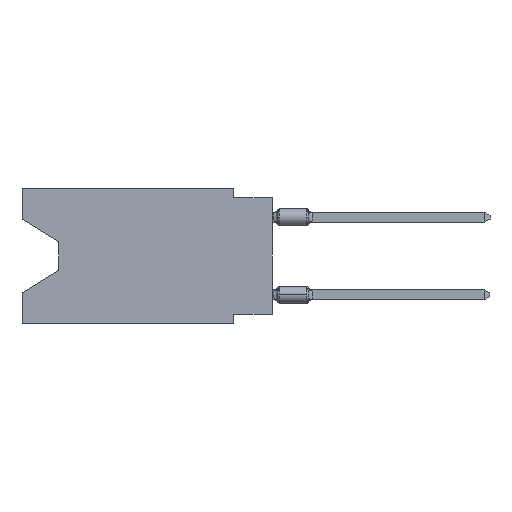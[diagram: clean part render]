
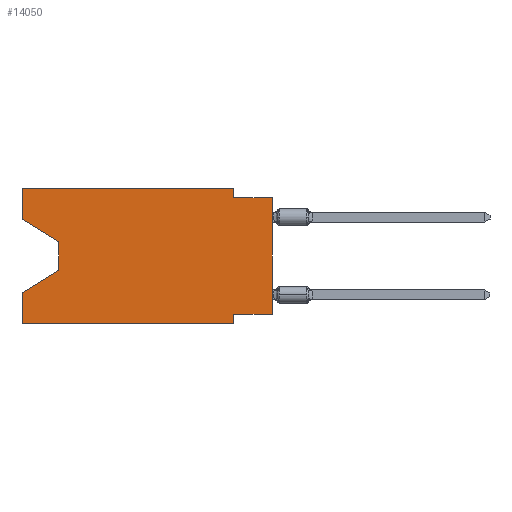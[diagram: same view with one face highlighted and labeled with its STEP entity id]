
A CAD part, left-side view. The second image highlights one B-rep face of the part: STEP entity #14050.
In plain terms, the highlighted planar face has unit normal (-1, 0, 0).
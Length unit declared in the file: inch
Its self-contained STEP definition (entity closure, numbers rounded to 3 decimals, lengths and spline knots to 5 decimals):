
#282 = CARTESIAN_POINT ( 'NONE',  ( 0., 0.1, -0.35 ) ) ;
#791 = FACE_OUTER_BOUND ( 'NONE', #29881, .T. ) ;
#947 = CARTESIAN_POINT ( 'NONE',  ( 0., 0.645, 0. ) ) ;
#1299 = LINE ( 'NONE', #24705, #29097 ) ;
#1441 = EDGE_CURVE ( 'NONE', #24950, #22444, #23115, .T. ) ;
#1586 = VERTEX_POINT ( 'NONE', #23418 ) ;
#1591 = CARTESIAN_POINT ( 'NONE',  ( 0., 0.645, 0. ) ) ;
#1623 = EDGE_CURVE ( 'NONE', #25172, #11600, #10286, .T. ) ;
#2054 = EDGE_CURVE ( 'NONE', #12673, #2710, #5565, .T. ) ;
#2333 = CARTESIAN_POINT ( 'NONE',  ( 0., 0.645, 0. ) ) ;
#2710 = VERTEX_POINT ( 'NONE', #29706 ) ;
#2850 = PLANE ( 'NONE',  #4351 ) ;
#3677 = DIRECTION ( 'NONE',  ( 0., -0.855, -0.519 ) ) ;
#4116 = CARTESIAN_POINT ( 'NONE',  ( 0., 0.645, -0.26975 ) ) ;
#4351 = AXIS2_PLACEMENT_3D ( 'NONE', #947, #19960, #12549 ) ;
#4737 = CARTESIAN_POINT ( 'NONE',  ( 0., 0.1, -0.325 ) ) ;
#5565 = LINE ( 'NONE', #22066, #23819 ) ;
#5657 = VERTEX_POINT ( 'NONE', #13763 ) ;
#5663 = DIRECTION ( 'NONE',  ( 0., 0., 1. ) ) ;
#6072 = CARTESIAN_POINT ( 'NONE',  ( 0., 0.645, -0.35 ) ) ;
#6188 = LINE ( 'NONE', #30512, #12170 ) ;
#7098 = ORIENTED_EDGE ( 'NONE', *, *, #16200, .F. ) ;
#7164 = LINE ( 'NONE', #14666, #29409 ) ;
#7353 = VECTOR ( 'NONE', #10313, 39.37008 ) ;
#7501 = LINE ( 'NONE', #282, #7353 ) ;
#7628 = DIRECTION ( 'NONE',  ( 0., 1., 0. ) ) ;
#7844 = VECTOR ( 'NONE', #5663, 39.37008 ) ;
#7947 = DIRECTION ( 'NONE',  ( 0., -1., 0. ) ) ;
#8277 = ORIENTED_EDGE ( 'NONE', *, *, #1441, .F. ) ;
#8848 = EDGE_CURVE ( 'NONE', #1586, #19466, #6188, .T. ) ;
#9090 = ORIENTED_EDGE ( 'NONE', *, *, #2054, .T. ) ;
#9843 = CARTESIAN_POINT ( 'NONE',  ( 0., 0.1, 0. ) ) ;
#10046 = LINE ( 'NONE', #19795, #7844 ) ;
#10286 = LINE ( 'NONE', #6072, #25681 ) ;
#10313 = DIRECTION ( 'NONE',  ( 0., 0., -1. ) ) ;
#11600 = VERTEX_POINT ( 'NONE', #29608 ) ;
#12170 = VECTOR ( 'NONE', #25810, 39.37008 ) ;
#12549 = DIRECTION ( 'NONE',  ( 0., 0., -1. ) ) ;
#12673 = VERTEX_POINT ( 'NONE', #26254 ) ;
#13719 = EDGE_CURVE ( 'NONE', #2710, #1586, #27368, .T. ) ;
#13763 = CARTESIAN_POINT ( 'NONE',  ( 0., 0., -0.025 ) ) ;
#14015 = VERTEX_POINT ( 'NONE', #4737 ) ;
#14050 = ADVANCED_FACE ( 'NONE', ( #791 ), #2850, .F. ) ;
#14138 = EDGE_CURVE ( 'NONE', #25172, #19466, #10046, .T. ) ;
#14520 = EDGE_CURVE ( 'NONE', #14015, #11600, #7501, .T. ) ;
#14666 = CARTESIAN_POINT ( 'NONE',  ( 0., 0., -0.325 ) ) ;
#14681 = DIRECTION ( 'NONE',  ( 0., 0., -1. ) ) ;
#14996 = CARTESIAN_POINT ( 'NONE',  ( 0., 0.1, 0. ) ) ;
#16200 = EDGE_CURVE ( 'NONE', #29581, #14015, #7164, .T. ) ;
#16208 = ORIENTED_EDGE ( 'NONE', *, *, #14138, .F. ) ;
#16277 = ORIENTED_EDGE ( 'NONE', *, *, #14520, .F. ) ;
#16588 = EDGE_CURVE ( 'NONE', #12673, #24950, #25491, .T. ) ;
#17918 = CARTESIAN_POINT ( 'NONE',  ( 0., 0.1, -0.025 ) ) ;
#18395 = VECTOR ( 'NONE', #23282, 39.37008 ) ;
#19290 = VERTEX_POINT ( 'NONE', #17918 ) ;
#19464 = ORIENTED_EDGE ( 'NONE', *, *, #13719, .T. ) ;
#19466 = VERTEX_POINT ( 'NONE', #4116 ) ;
#19795 = CARTESIAN_POINT ( 'NONE',  ( 0., 0.645, 0. ) ) ;
#19960 = DIRECTION ( 'NONE',  ( 1., 0., 0. ) ) ;
#20620 = CARTESIAN_POINT ( 'NONE',  ( 0., 0.645, 0. ) ) ;
#20698 = DIRECTION ( 'NONE',  ( 0., -1., 0. ) ) ;
#20966 = CARTESIAN_POINT ( 'NONE',  ( 0., 0.645, -0.35 ) ) ;
#21803 = LINE ( 'NONE', #9843, #30113 ) ;
#21891 = DIRECTION ( 'NONE',  ( 0., 0., -1. ) ) ;
#21896 = VECTOR ( 'NONE', #21891, 39.37008 ) ;
#22066 = CARTESIAN_POINT ( 'NONE',  ( 0., 0.645, -0.08025 ) ) ;
#22444 = VERTEX_POINT ( 'NONE', #14996 ) ;
#22517 = DIRECTION ( 'NONE',  ( 0., 0., 1. ) ) ;
#22568 = EDGE_CURVE ( 'NONE', #19290, #5657, #25241, .T. ) ;
#23115 = LINE ( 'NONE', #1591, #27716 ) ;
#23282 = DIRECTION ( 'NONE',  ( 0., 0., 1. ) ) ;
#23359 = EDGE_CURVE ( 'NONE', #29581, #5657, #1299, .T. ) ;
#23418 = CARTESIAN_POINT ( 'NONE',  ( 0., 0.55, -0.212 ) ) ;
#23819 = VECTOR ( 'NONE', #3677, 39.37008 ) ;
#24226 = CARTESIAN_POINT ( 'NONE',  ( 0., 0.55, -0.138 ) ) ;
#24258 = CARTESIAN_POINT ( 'NONE',  ( 0., 0., -0.325 ) ) ;
#24705 = CARTESIAN_POINT ( 'NONE',  ( 0., 0., 0. ) ) ;
#24950 = VERTEX_POINT ( 'NONE', #2333 ) ;
#24982 = EDGE_CURVE ( 'NONE', #22444, #19290, #21803, .T. ) ;
#25172 = VERTEX_POINT ( 'NONE', #20966 ) ;
#25241 = LINE ( 'NONE', #29639, #27585 ) ;
#25491 = LINE ( 'NONE', #20620, #18395 ) ;
#25681 = VECTOR ( 'NONE', #7947, 39.37008 ) ;
#25810 = DIRECTION ( 'NONE',  ( 0., 0.855, -0.519 ) ) ;
#26254 = CARTESIAN_POINT ( 'NONE',  ( 0., 0.645, -0.08025 ) ) ;
#26677 = ORIENTED_EDGE ( 'NONE', *, *, #8848, .T. ) ;
#26787 = ORIENTED_EDGE ( 'NONE', *, *, #24982, .F. ) ;
#26851 = ORIENTED_EDGE ( 'NONE', *, *, #1623, .T. ) ;
#27368 = LINE ( 'NONE', #24226, #21896 ) ;
#27585 = VECTOR ( 'NONE', #20698, 39.37008 ) ;
#27716 = VECTOR ( 'NONE', #30480, 39.37008 ) ;
#29097 = VECTOR ( 'NONE', #22517, 39.37008 ) ;
#29409 = VECTOR ( 'NONE', #7628, 39.37008 ) ;
#29581 = VERTEX_POINT ( 'NONE', #24258 ) ;
#29608 = CARTESIAN_POINT ( 'NONE',  ( 0., 0.1, -0.35 ) ) ;
#29639 = CARTESIAN_POINT ( 'NONE',  ( 0., 0., -0.025 ) ) ;
#29706 = CARTESIAN_POINT ( 'NONE',  ( 0., 0.55, -0.138 ) ) ;
#29837 = ORIENTED_EDGE ( 'NONE', *, *, #23359, .T. ) ;
#29881 = EDGE_LOOP ( 'NONE', ( #9090, #19464, #26677, #16208, #26851, #16277, #7098, #29837, #30887, #26787, #8277, #30735 ) ) ;
#30113 = VECTOR ( 'NONE', #14681, 39.37008 ) ;
#30480 = DIRECTION ( 'NONE',  ( 0., -1., 0. ) ) ;
#30512 = CARTESIAN_POINT ( 'NONE',  ( 0., 0.55, -0.212 ) ) ;
#30735 = ORIENTED_EDGE ( 'NONE', *, *, #16588, .F. ) ;
#30887 = ORIENTED_EDGE ( 'NONE', *, *, #22568, .F. ) ;
